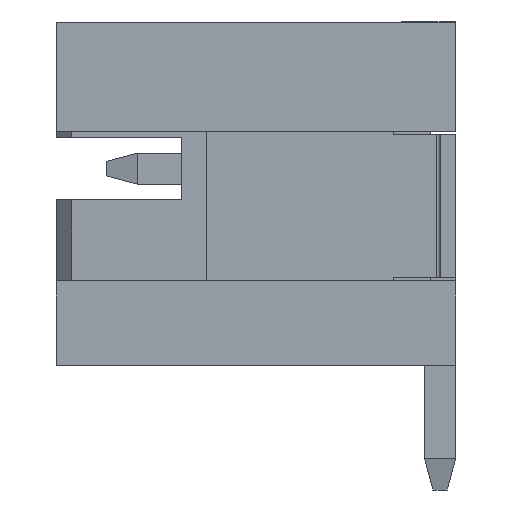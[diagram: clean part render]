
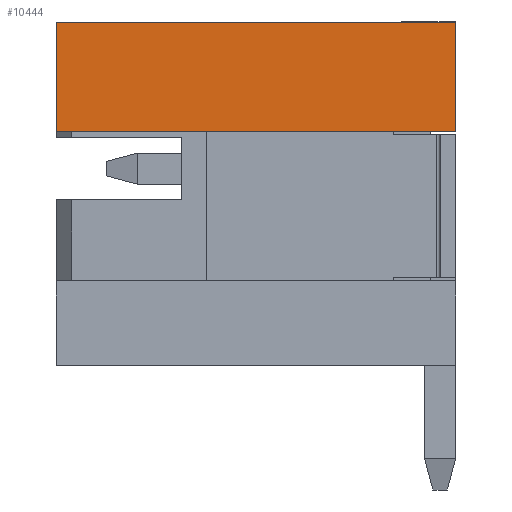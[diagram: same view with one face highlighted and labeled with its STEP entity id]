
A CAD part, left-side view. The second image highlights one B-rep face of the part: STEP entity #10444.
In plain terms, the highlighted planar face has unit normal (-1, 0, 0).
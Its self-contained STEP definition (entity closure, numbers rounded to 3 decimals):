
#560 = DIRECTION ( 'NONE',  ( 1., 0., 0. ) ) ;
#738 = ORIENTED_EDGE ( 'NONE', *, *, #4558, .F. ) ;
#787 = EDGE_CURVE ( 'NONE', #4195, #4926, #12363, .T. ) ;
#1140 = VECTOR ( 'NONE', #9895, 1000. ) ;
#1175 = DIRECTION ( 'NONE',  ( 0., 1., 0. ) ) ;
#1582 = VERTEX_POINT ( 'NONE', #10026 ) ;
#2865 = LINE ( 'NONE', #6305, #11936 ) ;
#3142 = CARTESIAN_POINT ( 'NONE',  ( -3., 0., 2.35 ) ) ;
#3740 = ORIENTED_EDGE ( 'NONE', *, *, #787, .F. ) ;
#4054 = EDGE_CURVE ( 'NONE', #1582, #6071, #9749, .T. ) ;
#4089 = CARTESIAN_POINT ( 'NONE',  ( -3., 0., 0.6 ) ) ;
#4195 = VERTEX_POINT ( 'NONE', #6137 ) ;
#4558 = EDGE_CURVE ( 'NONE', #4926, #1582, #8186, .T. ) ;
#4582 = EDGE_LOOP ( 'NONE', ( #6035, #738, #3740, #7333 ) ) ;
#4676 = AXIS2_PLACEMENT_3D ( 'NONE', #6346, #560, #10311 ) ;
#4926 = VERTEX_POINT ( 'NONE', #8197 ) ;
#6035 = ORIENTED_EDGE ( 'NONE', *, *, #4054, .F. ) ;
#6071 = VERTEX_POINT ( 'NONE', #9564 ) ;
#6137 = CARTESIAN_POINT ( 'NONE',  ( -3., 0., 2.35 ) ) ;
#6305 = CARTESIAN_POINT ( 'NONE',  ( -3., 6.4, 2.35 ) ) ;
#6346 = CARTESIAN_POINT ( 'NONE',  ( -3., 0., 0. ) ) ;
#7207 = DIRECTION ( 'NONE',  ( 0., -1., 0. ) ) ;
#7333 = ORIENTED_EDGE ( 'NONE', *, *, #12559, .F. ) ;
#8186 = LINE ( 'NONE', #4089, #8656 ) ;
#8197 = CARTESIAN_POINT ( 'NONE',  ( -3., 0., 0.6 ) ) ;
#8656 = VECTOR ( 'NONE', #1175, 1000. ) ;
#9564 = CARTESIAN_POINT ( 'NONE',  ( -3., 6.4, 2.35 ) ) ;
#9732 = VECTOR ( 'NONE', #11954, 1000. ) ;
#9749 = LINE ( 'NONE', #11013, #1140 ) ;
#9895 = DIRECTION ( 'NONE',  ( 0., 0., 1. ) ) ;
#10026 = CARTESIAN_POINT ( 'NONE',  ( -3., 6.4, 0.6 ) ) ;
#10311 = DIRECTION ( 'NONE',  ( 0., 0., -1. ) ) ;
#10444 = ADVANCED_FACE ( 'NONE', ( #11305 ), #11295, .F. ) ;
#11013 = CARTESIAN_POINT ( 'NONE',  ( -3., 6.4, 2.35 ) ) ;
#11295 = PLANE ( 'NONE',  #4676 ) ;
#11305 = FACE_OUTER_BOUND ( 'NONE', #4582, .T. ) ;
#11936 = VECTOR ( 'NONE', #7207, 1000. ) ;
#11954 = DIRECTION ( 'NONE',  ( 0., 0., -1. ) ) ;
#12363 = LINE ( 'NONE', #3142, #9732 ) ;
#12559 = EDGE_CURVE ( 'NONE', #6071, #4195, #2865, .T. ) ;
